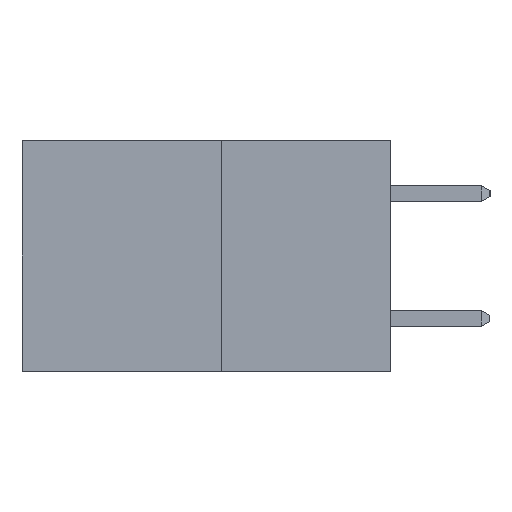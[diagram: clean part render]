
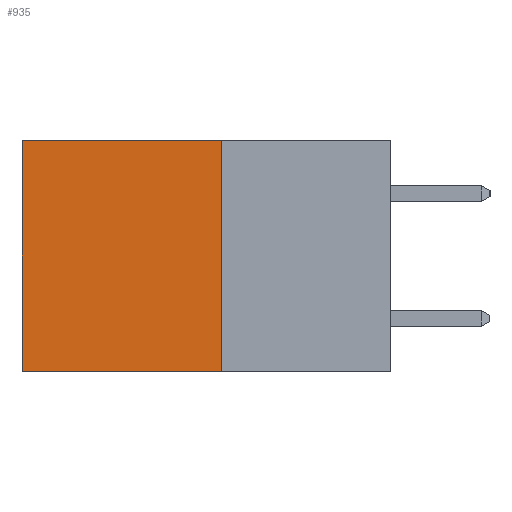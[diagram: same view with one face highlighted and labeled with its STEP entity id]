
A CAD part, left-side view. The second image highlights one B-rep face of the part: STEP entity #935.
In plain terms, the highlighted planar face has unit normal (-1, 0, 0).
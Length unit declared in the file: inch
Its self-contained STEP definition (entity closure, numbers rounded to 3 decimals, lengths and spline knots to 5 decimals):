
#372 = AXIS2_PLACEMENT_3D ( 'NONE', #13633, #18599, #10884 ) ;
#935 = ADVANCED_FACE ( 'NONE', ( #8694 ), #5527, .F. ) ;
#1498 = CARTESIAN_POINT ( 'NONE',  ( 0.277, 0.27, -0.37 ) ) ;
#1591 = CARTESIAN_POINT ( 'NONE',  ( 0.277, 0.27, -0.37 ) ) ;
#1697 = ORIENTED_EDGE ( 'NONE', *, *, #13505, .T. ) ;
#2429 = DIRECTION ( 'NONE',  ( 0., 1., 0. ) ) ;
#3131 = ORIENTED_EDGE ( 'NONE', *, *, #16346, .T. ) ;
#3809 = VECTOR ( 'NONE', #16373, 39.37008 ) ;
#4124 = VERTEX_POINT ( 'NONE', #11377 ) ;
#4399 = VECTOR ( 'NONE', #7387, 39.37008 ) ;
#5527 = PLANE ( 'NONE',  #372 ) ;
#5944 = CARTESIAN_POINT ( 'NONE',  ( 0.277, 0.27, 0. ) ) ;
#6228 = CARTESIAN_POINT ( 'NONE',  ( 0.277, 0.59, -0.37 ) ) ;
#6766 = CARTESIAN_POINT ( 'NONE',  ( 0.277, 0.59, -0.37 ) ) ;
#7149 = EDGE_CURVE ( 'NONE', #12110, #9634, #7779, .T. ) ;
#7165 = ORIENTED_EDGE ( 'NONE', *, *, #7416, .F. ) ;
#7387 = DIRECTION ( 'NONE',  ( 0., 1., 0. ) ) ;
#7416 = EDGE_CURVE ( 'NONE', #8433, #12110, #10499, .T. ) ;
#7779 = LINE ( 'NONE', #18432, #15044 ) ;
#8433 = VERTEX_POINT ( 'NONE', #12951 ) ;
#8694 = FACE_OUTER_BOUND ( 'NONE', #13022, .T. ) ;
#9168 = LINE ( 'NONE', #5944, #4399 ) ;
#9634 = VERTEX_POINT ( 'NONE', #6766 ) ;
#10499 = LINE ( 'NONE', #1498, #17798 ) ;
#10884 = DIRECTION ( 'NONE',  ( 0., 0., -1. ) ) ;
#11377 = CARTESIAN_POINT ( 'NONE',  ( 0.277, 0.59, 0. ) ) ;
#12110 = VERTEX_POINT ( 'NONE', #1591 ) ;
#12951 = CARTESIAN_POINT ( 'NONE',  ( 0.277, 0.27, 0. ) ) ;
#13022 = EDGE_LOOP ( 'NONE', ( #1697, #18549, #7165, #3131 ) ) ;
#13505 = EDGE_CURVE ( 'NONE', #4124, #9634, #14952, .T. ) ;
#13633 = CARTESIAN_POINT ( 'NONE',  ( 0.277, 0.27, -0.37 ) ) ;
#14952 = LINE ( 'NONE', #6228, #3809 ) ;
#15044 = VECTOR ( 'NONE', #2429, 39.37008 ) ;
#16346 = EDGE_CURVE ( 'NONE', #8433, #4124, #9168, .T. ) ;
#16373 = DIRECTION ( 'NONE',  ( 0., 0., -1. ) ) ;
#17565 = DIRECTION ( 'NONE',  ( 0., 0., -1. ) ) ;
#17798 = VECTOR ( 'NONE', #17565, 39.37008 ) ;
#18432 = CARTESIAN_POINT ( 'NONE',  ( 0.277, 0.27, -0.37 ) ) ;
#18549 = ORIENTED_EDGE ( 'NONE', *, *, #7149, .F. ) ;
#18599 = DIRECTION ( 'NONE',  ( 1., 0., 0. ) ) ;
